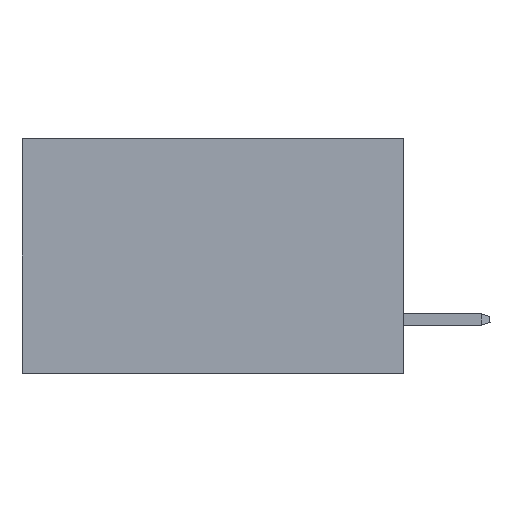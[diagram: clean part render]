
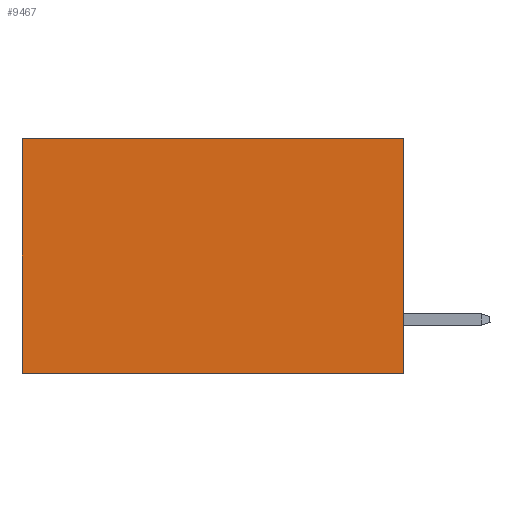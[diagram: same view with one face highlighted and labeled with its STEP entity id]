
A CAD part, left-side view. The second image highlights one B-rep face of the part: STEP entity #9467.
In plain terms, the highlighted planar face has unit normal (-1, 0, 0).
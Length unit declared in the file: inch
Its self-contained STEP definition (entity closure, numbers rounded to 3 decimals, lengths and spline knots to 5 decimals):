
#5093 = DIRECTION ( 'NONE',  ( 0., 0., -1. ) ) ;
#5783 = DIRECTION ( 'NONE',  ( 0., 0., -1. ) ) ;
#6018 = ORIENTED_EDGE ( 'NONE', *, *, #11010, .F. ) ;
#6616 = CARTESIAN_POINT ( 'NONE',  ( 0.2875, 0.6, 0. ) ) ;
#6681 = EDGE_LOOP ( 'NONE', ( #38735, #6018, #14684, #16692 ) ) ;
#7114 = LINE ( 'NONE', #20065, #37526 ) ;
#8728 = EDGE_CURVE ( 'NONE', #10693, #24591, #7114, .T. ) ;
#9467 = ADVANCED_FACE ( 'NONE', ( #18711 ), #15187, .F. ) ;
#10693 = VERTEX_POINT ( 'NONE', #21448 ) ;
#11010 = EDGE_CURVE ( 'NONE', #21687, #22009, #12416, .T. ) ;
#12416 = LINE ( 'NONE', #40620, #12588 ) ;
#12588 = VECTOR ( 'NONE', #33987, 39.37008 ) ;
#12888 = LINE ( 'NONE', #6616, #25248 ) ;
#14684 = ORIENTED_EDGE ( 'NONE', *, *, #34673, .F. ) ;
#15128 = CARTESIAN_POINT ( 'NONE',  ( 0.2875, 0., -0.37 ) ) ;
#15187 = PLANE ( 'NONE',  #38280 ) ;
#15710 = CARTESIAN_POINT ( 'NONE',  ( 0.2875, 0.6, 0. ) ) ;
#16692 = ORIENTED_EDGE ( 'NONE', *, *, #8728, .T. ) ;
#17184 = CARTESIAN_POINT ( 'NONE',  ( 0.2875, 0.6, -0.37 ) ) ;
#17810 = CARTESIAN_POINT ( 'NONE',  ( 0.2875, 0., 0. ) ) ;
#18497 = DIRECTION ( 'NONE',  ( 0., 0., -1. ) ) ;
#18711 = FACE_OUTER_BOUND ( 'NONE', #6681, .T. ) ;
#20065 = CARTESIAN_POINT ( 'NONE',  ( 0.2875, 0., 0. ) ) ;
#20339 = EDGE_CURVE ( 'NONE', #24591, #22009, #12888, .T. ) ;
#21448 = CARTESIAN_POINT ( 'NONE',  ( 0.2875, 0., 0. ) ) ;
#21644 = CARTESIAN_POINT ( 'NONE',  ( 0.2875, 0., 0. ) ) ;
#21687 = VERTEX_POINT ( 'NONE', #15128 ) ;
#22009 = VERTEX_POINT ( 'NONE', #17184 ) ;
#24591 = VERTEX_POINT ( 'NONE', #15710 ) ;
#25248 = VECTOR ( 'NONE', #5783, 39.37008 ) ;
#33947 = LINE ( 'NONE', #17810, #34485 ) ;
#33987 = DIRECTION ( 'NONE',  ( 0., 1., 0. ) ) ;
#34440 = DIRECTION ( 'NONE',  ( 1., 0., 0. ) ) ;
#34485 = VECTOR ( 'NONE', #5093, 39.37008 ) ;
#34673 = EDGE_CURVE ( 'NONE', #10693, #21687, #33947, .T. ) ;
#37526 = VECTOR ( 'NONE', #38895, 39.37008 ) ;
#38280 = AXIS2_PLACEMENT_3D ( 'NONE', #21644, #34440, #18497 ) ;
#38735 = ORIENTED_EDGE ( 'NONE', *, *, #20339, .T. ) ;
#38895 = DIRECTION ( 'NONE',  ( 0., 1., 0. ) ) ;
#40620 = CARTESIAN_POINT ( 'NONE',  ( 0.2875, 0., -0.37 ) ) ;
